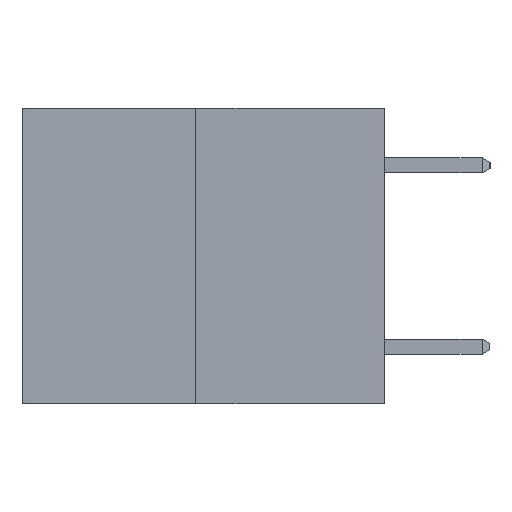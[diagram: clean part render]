
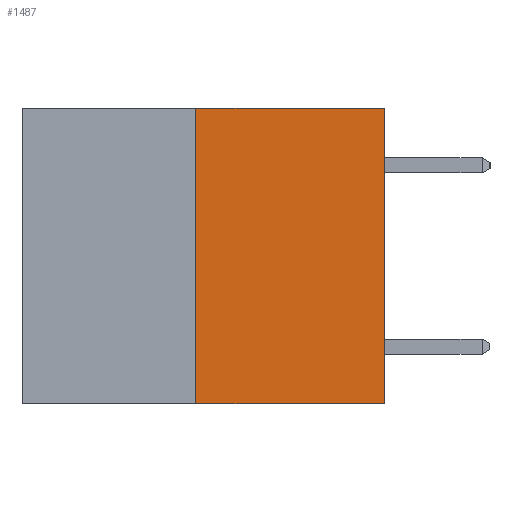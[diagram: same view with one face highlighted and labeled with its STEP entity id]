
A CAD part, left-side view. The second image highlights one B-rep face of the part: STEP entity #1487.
In plain terms, the highlighted planar face has unit normal (-1, 0, 0).
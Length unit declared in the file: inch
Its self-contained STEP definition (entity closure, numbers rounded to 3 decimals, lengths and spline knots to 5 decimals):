
#889 = DIRECTION ( 'NONE',  ( 0., -1., 0. ) ) ;
#1217 = VERTEX_POINT ( 'NONE', #3433 ) ;
#1299 = LINE ( 'NONE', #5002, #2472 ) ;
#1487 = ADVANCED_FACE ( 'NONE', ( #6187 ), #3763, .F. ) ;
#2472 = VECTOR ( 'NONE', #4128, 39.37008 ) ;
#2853 = CARTESIAN_POINT ( 'NONE',  ( 0., 0.6, 0. ) ) ;
#3062 = EDGE_CURVE ( 'NONE', #3271, #7988, #9480, .T. ) ;
#3271 = VERTEX_POINT ( 'NONE', #9149 ) ;
#3433 = CARTESIAN_POINT ( 'NONE',  ( 0., 0., -0.49 ) ) ;
#3718 = EDGE_CURVE ( 'NONE', #7988, #4765, #1299, .T. ) ;
#3763 = PLANE ( 'NONE',  #11612 ) ;
#4128 = DIRECTION ( 'NONE',  ( 0., -1., 0. ) ) ;
#4200 = VECTOR ( 'NONE', #8669, 39.37008 ) ;
#4765 = VERTEX_POINT ( 'NONE', #8835 ) ;
#5002 = CARTESIAN_POINT ( 'NONE',  ( 0., 0.6, 0. ) ) ;
#5133 = EDGE_LOOP ( 'NONE', ( #10115, #10497, #8908, #5178 ) ) ;
#5178 = ORIENTED_EDGE ( 'NONE', *, *, #3718, .F. ) ;
#5771 = DIRECTION ( 'NONE',  ( 1., 0., 0. ) ) ;
#6187 = FACE_OUTER_BOUND ( 'NONE', #5133, .T. ) ;
#6811 = EDGE_CURVE ( 'NONE', #1217, #4765, #10461, .T. ) ;
#7424 = CARTESIAN_POINT ( 'NONE',  ( 0., 0.6, -0.49 ) ) ;
#7709 = CARTESIAN_POINT ( 'NONE',  ( 0., 0., 0. ) ) ;
#7717 = EDGE_CURVE ( 'NONE', #3271, #1217, #12093, .T. ) ;
#7830 = CARTESIAN_POINT ( 'NONE',  ( 0., 0.312, -0.49 ) ) ;
#7988 = VERTEX_POINT ( 'NONE', #10873 ) ;
#8669 = DIRECTION ( 'NONE',  ( 0., 0., 1. ) ) ;
#8835 = CARTESIAN_POINT ( 'NONE',  ( 0., 0., 0. ) ) ;
#8908 = ORIENTED_EDGE ( 'NONE', *, *, #6811, .T. ) ;
#8973 = VECTOR ( 'NONE', #889, 39.37008 ) ;
#9149 = CARTESIAN_POINT ( 'NONE',  ( 0., 0.312, -0.49 ) ) ;
#9431 = DIRECTION ( 'NONE',  ( 0., 0., -1. ) ) ;
#9480 = LINE ( 'NONE', #7830, #10516 ) ;
#9729 = DIRECTION ( 'NONE',  ( 0., 0., 1. ) ) ;
#10115 = ORIENTED_EDGE ( 'NONE', *, *, #3062, .F. ) ;
#10461 = LINE ( 'NONE', #7709, #4200 ) ;
#10497 = ORIENTED_EDGE ( 'NONE', *, *, #7717, .T. ) ;
#10516 = VECTOR ( 'NONE', #9729, 39.37008 ) ;
#10873 = CARTESIAN_POINT ( 'NONE',  ( 0., 0.312, 0. ) ) ;
#11612 = AXIS2_PLACEMENT_3D ( 'NONE', #2853, #5771, #9431 ) ;
#12093 = LINE ( 'NONE', #7424, #8973 ) ;
